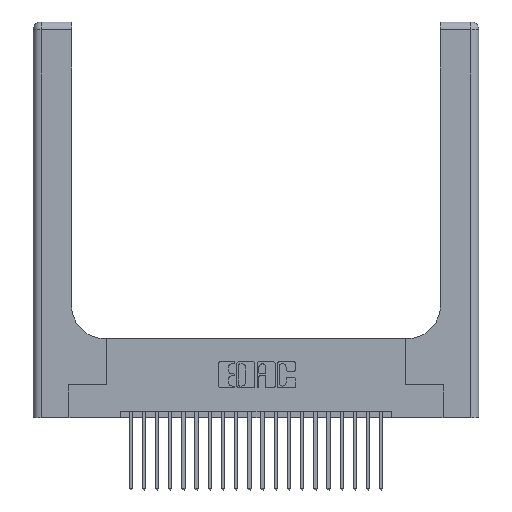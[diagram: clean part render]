
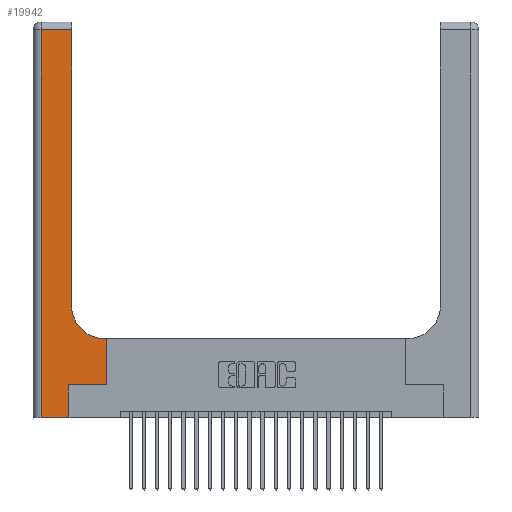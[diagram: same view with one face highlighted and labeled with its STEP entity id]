
A CAD part, top view. The second image highlights one B-rep face of the part: STEP entity #19942.
In plain terms, the highlighted planar face has unit normal (0, 0, 1).
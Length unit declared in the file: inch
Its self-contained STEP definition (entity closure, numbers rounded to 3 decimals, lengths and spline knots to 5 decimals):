
#255 = LINE ( 'NONE', #1046, #13976 ) ;
#346 = ORIENTED_EDGE ( 'NONE', *, *, #1980, .T. ) ;
#418 = VECTOR ( 'NONE', #6628, 39.37008 ) ;
#1046 = CARTESIAN_POINT ( 'NONE',  ( 0.2915, 0.6, 0.37 ) ) ;
#1157 = CARTESIAN_POINT ( 'NONE',  ( 0., 3., 0.37 ) ) ;
#1347 = VERTEX_POINT ( 'NONE', #16725 ) ;
#1369 = DIRECTION ( 'NONE',  ( 1., 0., 0. ) ) ;
#1946 = VERTEX_POINT ( 'NONE', #8286 ) ;
#1980 = EDGE_CURVE ( 'NONE', #5439, #16154, #3233, .T. ) ;
#2053 = ORIENTED_EDGE ( 'NONE', *, *, #20652, .T. ) ;
#3087 = LINE ( 'NONE', #23425, #12486 ) ;
#3233 = CIRCLE ( 'NONE', #14538, 0.25 ) ;
#4031 = EDGE_CURVE ( 'NONE', #16154, #1946, #22506, .T. ) ;
#4040 = ORIENTED_EDGE ( 'NONE', *, *, #11532, .T. ) ;
#4873 = DIRECTION ( 'NONE',  ( -1., 0., 0. ) ) ;
#5439 = VERTEX_POINT ( 'NONE', #18856 ) ;
#6258 = LINE ( 'NONE', #8149, #20432 ) ;
#6304 = ORIENTED_EDGE ( 'NONE', *, *, #4031, .T. ) ;
#6568 = DIRECTION ( 'NONE',  ( 0., -1., 0. ) ) ;
#6628 = DIRECTION ( 'NONE',  ( 0., 1., 0. ) ) ;
#7495 = CARTESIAN_POINT ( 'NONE',  ( 0.06, 2.94, 0.37 ) ) ;
#8100 = EDGE_CURVE ( 'NONE', #20670, #17312, #20126, .T. ) ;
#8149 = CARTESIAN_POINT ( 'NONE',  ( 0., 2.94, 0.37 ) ) ;
#8243 = EDGE_CURVE ( 'NONE', #23372, #11349, #12376, .T. ) ;
#8286 = CARTESIAN_POINT ( 'NONE',  ( 0.2915, 2.94, 0.37 ) ) ;
#8442 = DIRECTION ( 'NONE',  ( 0., 0., -1. ) ) ;
#8566 = DIRECTION ( 'NONE',  ( -1., 0., 0. ) ) ;
#8604 = DIRECTION ( 'NONE',  ( 0., 0., -1. ) ) ;
#8877 = DIRECTION ( 'NONE',  ( 0., 1., 0. ) ) ;
#9319 = CARTESIAN_POINT ( 'NONE',  ( 0.269, 0.25, 0.37 ) ) ;
#10017 = DIRECTION ( 'NONE',  ( -1., 0., 0. ) ) ;
#10856 = CARTESIAN_POINT ( 'NONE',  ( 0.2915, 3., 0.37 ) ) ;
#11349 = VERTEX_POINT ( 'NONE', #13298 ) ;
#11532 = EDGE_CURVE ( 'NONE', #14178, #1347, #19967, .T. ) ;
#11576 = EDGE_CURVE ( 'NONE', #17312, #5439, #255, .T. ) ;
#11733 = ORIENTED_EDGE ( 'NONE', *, *, #8100, .T. ) ;
#12152 = CARTESIAN_POINT ( 'NONE',  ( 0.06, 3., 0.37 ) ) ;
#12376 = LINE ( 'NONE', #21685, #22074 ) ;
#12486 = VECTOR ( 'NONE', #1369, 39.37008 ) ;
#12636 = CARTESIAN_POINT ( 'NONE',  ( 0.5585, 0.25, 0.37 ) ) ;
#13165 = CARTESIAN_POINT ( 'NONE',  ( 0.2915, 0.85, 0.37 ) ) ;
#13298 = CARTESIAN_POINT ( 'NONE',  ( 0.269, 0.25, 0.37 ) ) ;
#13976 = VECTOR ( 'NONE', #8566, 39.37008 ) ;
#14004 = ORIENTED_EDGE ( 'NONE', *, *, #22092, .T. ) ;
#14178 = VERTEX_POINT ( 'NONE', #7495 ) ;
#14538 = AXIS2_PLACEMENT_3D ( 'NONE', #19482, #8442, #21287 ) ;
#15227 = ORIENTED_EDGE ( 'NONE', *, *, #20204, .T. ) ;
#15313 = EDGE_LOOP ( 'NONE', ( #6304, #14004, #4040, #2053, #19770, #15227, #11733, #22010, #346 ) ) ;
#16078 = PLANE ( 'NONE',  #20766 ) ;
#16154 = VERTEX_POINT ( 'NONE', #13165 ) ;
#16715 = DIRECTION ( 'NONE',  ( 1., 0., 0. ) ) ;
#16725 = CARTESIAN_POINT ( 'NONE',  ( 0.06, 0., 0.37 ) ) ;
#17170 = VECTOR ( 'NONE', #21809, 39.37008 ) ;
#17312 = VERTEX_POINT ( 'NONE', #23739 ) ;
#17440 = VECTOR ( 'NONE', #16715, 39.37008 ) ;
#17729 = FACE_OUTER_BOUND ( 'NONE', #15313, .T. ) ;
#17819 = CARTESIAN_POINT ( 'NONE',  ( 0.269, 0., 0.37 ) ) ;
#18856 = CARTESIAN_POINT ( 'NONE',  ( 0.5415, 0.6, 0.37 ) ) ;
#19403 = VECTOR ( 'NONE', #6568, 39.37008 ) ;
#19482 = CARTESIAN_POINT ( 'NONE',  ( 0.5415, 0.85, 0.37 ) ) ;
#19589 = CARTESIAN_POINT ( 'NONE',  ( 0.5585, 0.25, 0.37 ) ) ;
#19770 = ORIENTED_EDGE ( 'NONE', *, *, #8243, .T. ) ;
#19942 = ADVANCED_FACE ( 'NONE', ( #17729 ), #16078, .F. ) ;
#19967 = LINE ( 'NONE', #12152, #19403 ) ;
#20126 = LINE ( 'NONE', #19589, #418 ) ;
#20204 = EDGE_CURVE ( 'NONE', #11349, #20670, #22198, .T. ) ;
#20432 = VECTOR ( 'NONE', #10017, 39.37008 ) ;
#20652 = EDGE_CURVE ( 'NONE', #1347, #23372, #3087, .T. ) ;
#20670 = VERTEX_POINT ( 'NONE', #12636 ) ;
#20766 = AXIS2_PLACEMENT_3D ( 'NONE', #1157, #8604, #4873 ) ;
#21287 = DIRECTION ( 'NONE',  ( 1., 0., 0. ) ) ;
#21685 = CARTESIAN_POINT ( 'NONE',  ( 0.269, 0., 0.37 ) ) ;
#21809 = DIRECTION ( 'NONE',  ( 0., 1., 0. ) ) ;
#22010 = ORIENTED_EDGE ( 'NONE', *, *, #11576, .T. ) ;
#22074 = VECTOR ( 'NONE', #8877, 39.37008 ) ;
#22092 = EDGE_CURVE ( 'NONE', #1946, #14178, #6258, .T. ) ;
#22198 = LINE ( 'NONE', #9319, #17440 ) ;
#22506 = LINE ( 'NONE', #10856, #17170 ) ;
#23372 = VERTEX_POINT ( 'NONE', #17819 ) ;
#23425 = CARTESIAN_POINT ( 'NONE',  ( 0., 0., 0.37 ) ) ;
#23739 = CARTESIAN_POINT ( 'NONE',  ( 0.5585, 0.6, 0.37 ) ) ;
